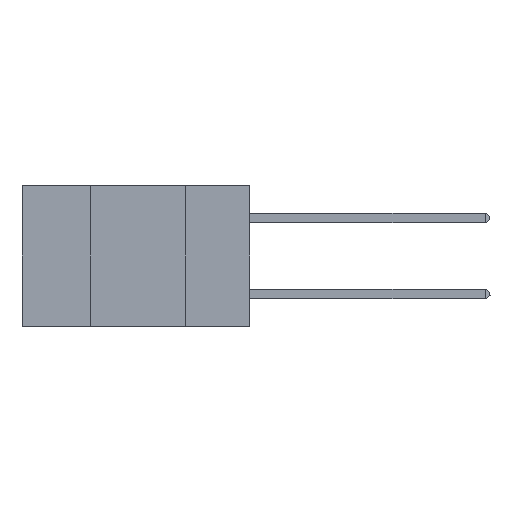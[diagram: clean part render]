
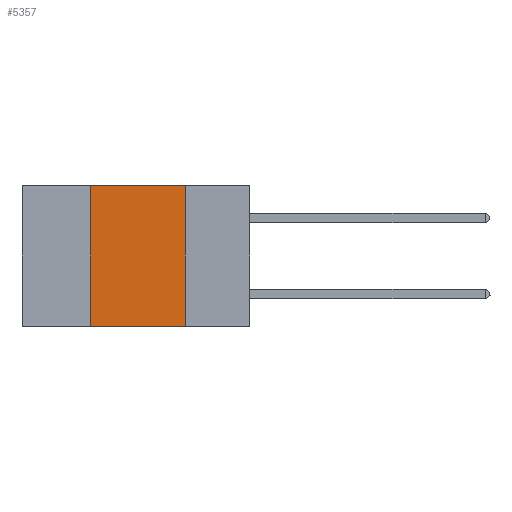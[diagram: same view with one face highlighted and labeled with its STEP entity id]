
A CAD part, left-side view. The second image highlights one B-rep face of the part: STEP entity #5357.
In plain terms, the highlighted planar face has unit normal (-1, 0, 0).
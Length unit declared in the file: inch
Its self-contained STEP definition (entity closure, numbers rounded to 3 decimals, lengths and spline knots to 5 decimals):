
#640 = CARTESIAN_POINT ( 'NONE',  ( 0., 0.17, 0. ) ) ;
#2157 = DIRECTION ( 'NONE',  ( 0., 0., 1. ) ) ;
#2184 = CARTESIAN_POINT ( 'NONE',  ( 0., 0.6, 0. ) ) ;
#2586 = CARTESIAN_POINT ( 'NONE',  ( 0., 0.42, 0. ) ) ;
#3050 = ORIENTED_EDGE ( 'NONE', *, *, #16106, .T. ) ;
#3231 = VECTOR ( 'NONE', #2157, 39.37008 ) ;
#3834 = VECTOR ( 'NONE', #10081, 39.37008 ) ;
#3915 = DIRECTION ( 'NONE',  ( 1., 0., 0. ) ) ;
#4153 = CARTESIAN_POINT ( 'NONE',  ( 0., 0.42, -0.37 ) ) ;
#5357 = ADVANCED_FACE ( 'NONE', ( #12970 ), #21316, .F. ) ;
#5416 = VERTEX_POINT ( 'NONE', #14423 ) ;
#8757 = EDGE_LOOP ( 'NONE', ( #13565, #15844, #22334, #3050 ) ) ;
#10081 = DIRECTION ( 'NONE',  ( 0., -1., 0. ) ) ;
#12524 = CARTESIAN_POINT ( 'NONE',  ( 0., 0.6, 0. ) ) ;
#12528 = DIRECTION ( 'NONE',  ( 0., 0., -1. ) ) ;
#12581 = AXIS2_PLACEMENT_3D ( 'NONE', #2184, #3915, #17861 ) ;
#12970 = FACE_OUTER_BOUND ( 'NONE', #8757, .T. ) ;
#13269 = LINE ( 'NONE', #13918, #18199 ) ;
#13565 = ORIENTED_EDGE ( 'NONE', *, *, #14194, .F. ) ;
#13918 = CARTESIAN_POINT ( 'NONE',  ( 0., 0.6, -0.37 ) ) ;
#14194 = EDGE_CURVE ( 'NONE', #22060, #5416, #17391, .T. ) ;
#14423 = CARTESIAN_POINT ( 'NONE',  ( 0., 0.17, -0.37 ) ) ;
#15004 = LINE ( 'NONE', #12524, #3834 ) ;
#15193 = VECTOR ( 'NONE', #12528, 39.37008 ) ;
#15844 = ORIENTED_EDGE ( 'NONE', *, *, #20529, .F. ) ;
#16019 = VERTEX_POINT ( 'NONE', #2586 ) ;
#16106 = EDGE_CURVE ( 'NONE', #22041, #5416, #13269, .T. ) ;
#16285 = CARTESIAN_POINT ( 'NONE',  ( 0., 0.17, 0. ) ) ;
#16558 = LINE ( 'NONE', #19451, #3231 ) ;
#17391 = LINE ( 'NONE', #16285, #15193 ) ;
#17861 = DIRECTION ( 'NONE',  ( 0., 0., -1. ) ) ;
#18199 = VECTOR ( 'NONE', #19564, 39.37008 ) ;
#19451 = CARTESIAN_POINT ( 'NONE',  ( 0., 0.42, 0. ) ) ;
#19564 = DIRECTION ( 'NONE',  ( 0., -1., 0. ) ) ;
#20529 = EDGE_CURVE ( 'NONE', #16019, #22060, #15004, .T. ) ;
#21316 = PLANE ( 'NONE',  #12581 ) ;
#22041 = VERTEX_POINT ( 'NONE', #4153 ) ;
#22060 = VERTEX_POINT ( 'NONE', #640 ) ;
#22334 = ORIENTED_EDGE ( 'NONE', *, *, #22474, .F. ) ;
#22474 = EDGE_CURVE ( 'NONE', #22041, #16019, #16558, .T. ) ;
